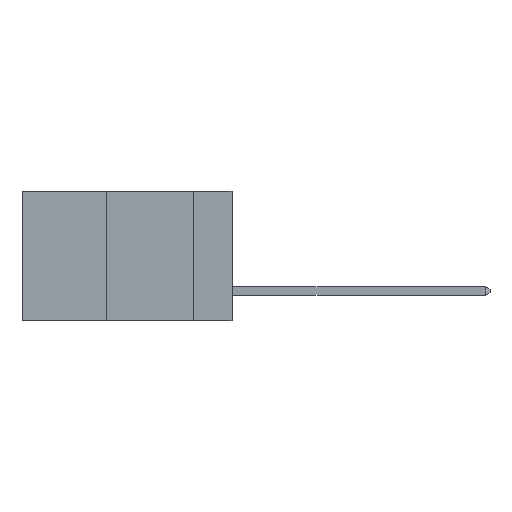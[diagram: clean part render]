
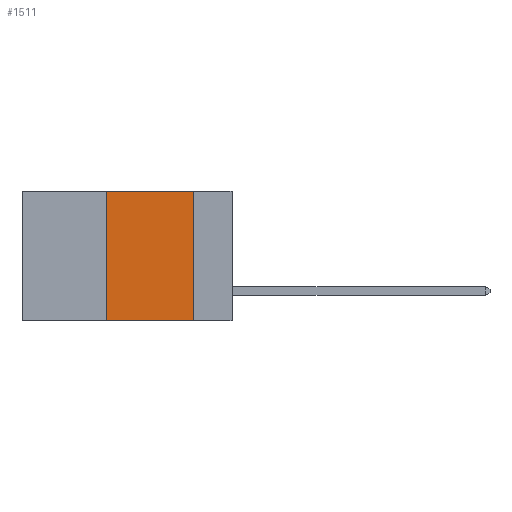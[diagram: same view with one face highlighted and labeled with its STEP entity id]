
A CAD part, left-side view. The second image highlights one B-rep face of the part: STEP entity #1511.
In plain terms, the highlighted planar face has unit normal (-1, 0, 0).
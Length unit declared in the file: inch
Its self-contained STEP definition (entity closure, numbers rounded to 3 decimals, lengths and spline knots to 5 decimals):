
#836 = EDGE_CURVE ( 'NONE', #11082, #10503, #9090, .T. ) ;
#1511 = ADVANCED_FACE ( 'NONE', ( #4862 ), #3515, .F. ) ;
#2398 = DIRECTION ( 'NONE',  ( 0., -1., 0. ) ) ;
#3359 = CARTESIAN_POINT ( 'NONE',  ( 0., 0.6, 0. ) ) ;
#3397 = LINE ( 'NONE', #8301, #3707 ) ;
#3515 = PLANE ( 'NONE',  #8357 ) ;
#3675 = ORIENTED_EDGE ( 'NONE', *, *, #9593, .F. ) ;
#3707 = VECTOR ( 'NONE', #2398, 39.37008 ) ;
#3889 = EDGE_CURVE ( 'NONE', #8799, #10503, #12343, .T. ) ;
#4257 = ORIENTED_EDGE ( 'NONE', *, *, #3889, .T. ) ;
#4715 = DIRECTION ( 'NONE',  ( 0., 0., 1. ) ) ;
#4862 = FACE_OUTER_BOUND ( 'NONE', #6059, .T. ) ;
#4881 = CARTESIAN_POINT ( 'NONE',  ( 0., 0.6, -0.37 ) ) ;
#5038 = DIRECTION ( 'NONE',  ( 1., 0., 0. ) ) ;
#5537 = VERTEX_POINT ( 'NONE', #6957 ) ;
#5713 = CARTESIAN_POINT ( 'NONE',  ( 0., 0.36, 0. ) ) ;
#5757 = LINE ( 'NONE', #5713, #10905 ) ;
#5905 = DIRECTION ( 'NONE',  ( 0., -1., 0. ) ) ;
#6059 = EDGE_LOOP ( 'NONE', ( #10686, #11234, #3675, #4257 ) ) ;
#6091 = CARTESIAN_POINT ( 'NONE',  ( 0., 0.11, -0.37 ) ) ;
#6650 = DIRECTION ( 'NONE',  ( 0., 0., -1. ) ) ;
#6677 = VECTOR ( 'NONE', #8411, 39.37008 ) ;
#6957 = CARTESIAN_POINT ( 'NONE',  ( 0., 0.36, 0. ) ) ;
#7946 = VECTOR ( 'NONE', #5905, 39.37008 ) ;
#8301 = CARTESIAN_POINT ( 'NONE',  ( 0., 0.6, 0. ) ) ;
#8357 = AXIS2_PLACEMENT_3D ( 'NONE', #3359, #5038, #6650 ) ;
#8411 = DIRECTION ( 'NONE',  ( 0., 0., -1. ) ) ;
#8684 = EDGE_CURVE ( 'NONE', #5537, #11082, #3397, .T. ) ;
#8799 = VERTEX_POINT ( 'NONE', #10227 ) ;
#9090 = LINE ( 'NONE', #12089, #6677 ) ;
#9593 = EDGE_CURVE ( 'NONE', #8799, #5537, #5757, .T. ) ;
#10227 = CARTESIAN_POINT ( 'NONE',  ( 0., 0.36, -0.37 ) ) ;
#10423 = CARTESIAN_POINT ( 'NONE',  ( 0., 0.11, 0. ) ) ;
#10503 = VERTEX_POINT ( 'NONE', #6091 ) ;
#10686 = ORIENTED_EDGE ( 'NONE', *, *, #836, .F. ) ;
#10905 = VECTOR ( 'NONE', #4715, 39.37008 ) ;
#11082 = VERTEX_POINT ( 'NONE', #10423 ) ;
#11234 = ORIENTED_EDGE ( 'NONE', *, *, #8684, .F. ) ;
#12089 = CARTESIAN_POINT ( 'NONE',  ( 0., 0.11, 0. ) ) ;
#12343 = LINE ( 'NONE', #4881, #7946 ) ;
